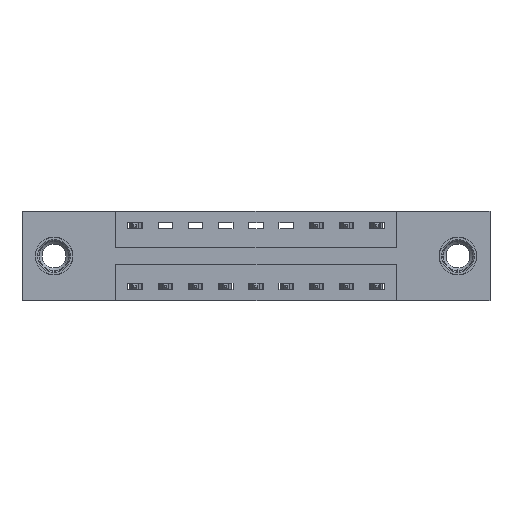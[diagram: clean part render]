
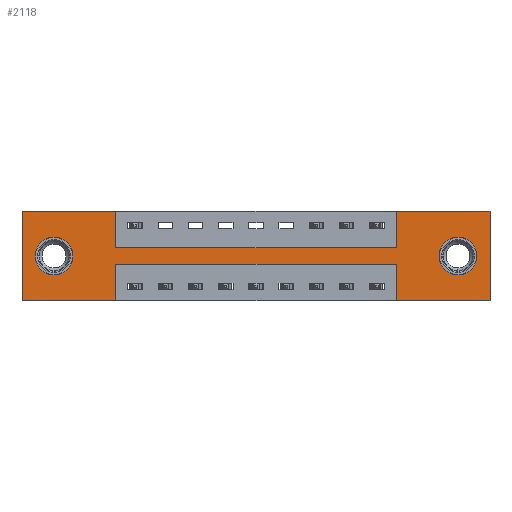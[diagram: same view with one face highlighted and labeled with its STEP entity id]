
A CAD part, front view. The second image highlights one B-rep face of the part: STEP entity #2118.
In plain terms, the highlighted planar face has unit normal (0, -1, 0).
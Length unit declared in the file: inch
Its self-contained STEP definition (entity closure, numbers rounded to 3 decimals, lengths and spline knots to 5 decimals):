
#57 = CARTESIAN_POINT ( 'NONE',  ( 1.935, 0., 0. ) ) ;
#127 = VECTOR ( 'NONE', #6239, 39.37008 ) ;
#150 = DIRECTION ( 'NONE',  ( 0., 1., 0. ) ) ;
#195 = VERTEX_POINT ( 'NONE', #1188 ) ;
#351 = DIRECTION ( 'NONE',  ( 0., 1., 0. ) ) ;
#354 = EDGE_CURVE ( 'NONE', #7185, #7598, #6876, .T. ) ;
#405 = FACE_BOUND ( 'NONE', #10598, .T. ) ;
#588 = ORIENTED_EDGE ( 'NONE', *, *, #4036, .T. ) ;
#617 = DIRECTION ( 'NONE',  ( -1., 0., 0. ) ) ;
#630 = VECTOR ( 'NONE', #2330, 39.37008 ) ;
#754 = VECTOR ( 'NONE', #3421, 39.37008 ) ;
#954 = CARTESIAN_POINT ( 'NONE',  ( 1.5475, 0., -0.37 ) ) ;
#1026 = LINE ( 'NONE', #11291, #754 ) ;
#1104 = ORIENTED_EDGE ( 'NONE', *, *, #2130, .F. ) ;
#1188 = CARTESIAN_POINT ( 'NONE',  ( 1.935, 0., -0.37 ) ) ;
#1241 = VECTOR ( 'NONE', #8316, 39.37008 ) ;
#1261 = VECTOR ( 'NONE', #5173, 39.37008 ) ;
#1417 = CARTESIAN_POINT ( 'NONE',  ( 1.8025, 0., -0.263 ) ) ;
#1550 = EDGE_CURVE ( 'NONE', #11316, #2201, #3587, .T. ) ;
#1667 = CARTESIAN_POINT ( 'NONE',  ( 0.3875, 0., 0. ) ) ;
#1832 = ORIENTED_EDGE ( 'NONE', *, *, #4395, .F. ) ;
#1946 = VECTOR ( 'NONE', #5117, 39.37008 ) ;
#2118 = ADVANCED_FACE ( 'NONE', ( #405, #2480, #7089 ), #8846, .T. ) ;
#2130 = EDGE_CURVE ( 'NONE', #7598, #3999, #9184, .T. ) ;
#2134 = VECTOR ( 'NONE', #10495, 39.37008 ) ;
#2201 = VERTEX_POINT ( 'NONE', #4592 ) ;
#2222 = CARTESIAN_POINT ( 'NONE',  ( 1.8025, 0., -0.107 ) ) ;
#2330 = DIRECTION ( 'NONE',  ( 1., 0., 0. ) ) ;
#2353 = CIRCLE ( 'NONE', #6170, 0.078 ) ;
#2410 = ORIENTED_EDGE ( 'NONE', *, *, #9981, .F. ) ;
#2420 = CIRCLE ( 'NONE', #6364, 0.078 ) ;
#2474 = DIRECTION ( 'NONE',  ( 1., 0., 0. ) ) ;
#2480 = FACE_BOUND ( 'NONE', #8097, .T. ) ;
#2612 = CARTESIAN_POINT ( 'NONE',  ( 0.3875, 0., -0.15 ) ) ;
#2656 = ORIENTED_EDGE ( 'NONE', *, *, #7369, .T. ) ;
#2743 = DIRECTION ( 'NONE',  ( 0., 1., 0. ) ) ;
#2757 = EDGE_CURVE ( 'NONE', #5667, #10404, #11383, .T. ) ;
#2888 = ORIENTED_EDGE ( 'NONE', *, *, #354, .F. ) ;
#2892 = CARTESIAN_POINT ( 'NONE',  ( 1.5475, 0., 0. ) ) ;
#2978 = VERTEX_POINT ( 'NONE', #9190 ) ;
#3146 = DIRECTION ( 'NONE',  ( 0., 0., 1. ) ) ;
#3162 = VERTEX_POINT ( 'NONE', #3290 ) ;
#3273 = ORIENTED_EDGE ( 'NONE', *, *, #5122, .F. ) ;
#3290 = CARTESIAN_POINT ( 'NONE',  ( 0.3875, 0., 0. ) ) ;
#3421 = DIRECTION ( 'NONE',  ( 0., 0., -1. ) ) ;
#3515 = AXIS2_PLACEMENT_3D ( 'NONE', #7959, #2743, #8843 ) ;
#3536 = EDGE_CURVE ( 'NONE', #6486, #195, #6248, .T. ) ;
#3587 = LINE ( 'NONE', #4345, #1241 ) ;
#3605 = DIRECTION ( 'NONE',  ( 0., 1., 0. ) ) ;
#3626 = CARTESIAN_POINT ( 'NONE',  ( 0., 0., -0.37 ) ) ;
#3650 = LINE ( 'NONE', #5843, #8001 ) ;
#3741 = DIRECTION ( 'NONE',  ( 0., 0., -1. ) ) ;
#3999 = VERTEX_POINT ( 'NONE', #6162 ) ;
#4036 = EDGE_CURVE ( 'NONE', #7563, #2978, #7182, .T. ) ;
#4074 = CARTESIAN_POINT ( 'NONE',  ( 1.5475, 0., -0.22 ) ) ;
#4232 = CARTESIAN_POINT ( 'NONE',  ( 0.3875, 0., -0.15 ) ) ;
#4345 = CARTESIAN_POINT ( 'NONE',  ( 0., 0., 0. ) ) ;
#4395 = EDGE_CURVE ( 'NONE', #2201, #3162, #5953, .T. ) ;
#4423 = LINE ( 'NONE', #7824, #2134 ) ;
#4437 = EDGE_CURVE ( 'NONE', #3999, #5343, #1026, .T. ) ;
#4473 = CARTESIAN_POINT ( 'NONE',  ( 0.3875, 0., -0.22 ) ) ;
#4592 = CARTESIAN_POINT ( 'NONE',  ( 0., 0., 0. ) ) ;
#5058 = ORIENTED_EDGE ( 'NONE', *, *, #6924, .F. ) ;
#5116 = CARTESIAN_POINT ( 'NONE',  ( 1.5475, 0., -0.15 ) ) ;
#5117 = DIRECTION ( 'NONE',  ( 1., 0., 0. ) ) ;
#5122 = EDGE_CURVE ( 'NONE', #195, #7185, #3650, .T. ) ;
#5173 = DIRECTION ( 'NONE',  ( 0., 0., -1. ) ) ;
#5343 = VERTEX_POINT ( 'NONE', #6151 ) ;
#5368 = DIRECTION ( 'NONE',  ( 0., 0., -1. ) ) ;
#5387 = AXIS2_PLACEMENT_3D ( 'NONE', #3626, #10645, #5368 ) ;
#5389 = CARTESIAN_POINT ( 'NONE',  ( 1.8025, 0., -0.185 ) ) ;
#5522 = DIRECTION ( 'NONE',  ( 0., 0., 1. ) ) ;
#5542 = AXIS2_PLACEMENT_3D ( 'NONE', #5389, #150, #6262 ) ;
#5581 = CARTESIAN_POINT ( 'NONE',  ( 1.8025, 0., -0.185 ) ) ;
#5597 = VECTOR ( 'NONE', #5522, 39.37008 ) ;
#5667 = VERTEX_POINT ( 'NONE', #1417 ) ;
#5743 = CARTESIAN_POINT ( 'NONE',  ( 0., 0., -0.37 ) ) ;
#5798 = CARTESIAN_POINT ( 'NONE',  ( 0.1325, 0., -0.263 ) ) ;
#5843 = CARTESIAN_POINT ( 'NONE',  ( 0., 0., -0.37 ) ) ;
#5921 = EDGE_CURVE ( 'NONE', #5343, #11316, #4423, .T. ) ;
#5953 = LINE ( 'NONE', #10357, #7999 ) ;
#6151 = CARTESIAN_POINT ( 'NONE',  ( 0.3875, 0., -0.37 ) ) ;
#6162 = CARTESIAN_POINT ( 'NONE',  ( 0.3875, 0., -0.22 ) ) ;
#6170 = AXIS2_PLACEMENT_3D ( 'NONE', #8825, #3605, #9724 ) ;
#6239 = DIRECTION ( 'NONE',  ( -1., 0., 0. ) ) ;
#6248 = LINE ( 'NONE', #9023, #10390 ) ;
#6262 = DIRECTION ( 'NONE',  ( 0., 0., -1. ) ) ;
#6364 = AXIS2_PLACEMENT_3D ( 'NONE', #5581, #351, #6455 ) ;
#6455 = DIRECTION ( 'NONE',  ( 0., 0., -1. ) ) ;
#6486 = VERTEX_POINT ( 'NONE', #57 ) ;
#6597 = VECTOR ( 'NONE', #3146, 39.37008 ) ;
#6793 = ORIENTED_EDGE ( 'NONE', *, *, #4437, .F. ) ;
#6876 = LINE ( 'NONE', #8363, #6597 ) ;
#6924 = EDGE_CURVE ( 'NONE', #8419, #6486, #7322, .T. ) ;
#7058 = ORIENTED_EDGE ( 'NONE', *, *, #9382, .F. ) ;
#7089 = FACE_OUTER_BOUND ( 'NONE', #10559, .T. ) ;
#7182 = CIRCLE ( 'NONE', #3515, 0.078 ) ;
#7185 = VERTEX_POINT ( 'NONE', #954 ) ;
#7322 = LINE ( 'NONE', #11103, #630 ) ;
#7369 = EDGE_CURVE ( 'NONE', #10404, #5667, #2420, .T. ) ;
#7563 = VERTEX_POINT ( 'NONE', #5798 ) ;
#7598 = VERTEX_POINT ( 'NONE', #4074 ) ;
#7707 = VERTEX_POINT ( 'NONE', #5116 ) ;
#7773 = VERTEX_POINT ( 'NONE', #2612 ) ;
#7824 = CARTESIAN_POINT ( 'NONE',  ( 0., 0., -0.37 ) ) ;
#7959 = CARTESIAN_POINT ( 'NONE',  ( 0.1325, 0., -0.185 ) ) ;
#7999 = VECTOR ( 'NONE', #2474, 39.37008 ) ;
#8001 = VECTOR ( 'NONE', #617, 39.37008 ) ;
#8097 = EDGE_LOOP ( 'NONE', ( #9697, #588 ) ) ;
#8316 = DIRECTION ( 'NONE',  ( 0., 0., 1. ) ) ;
#8363 = CARTESIAN_POINT ( 'NONE',  ( 1.5475, 0., -0.37 ) ) ;
#8419 = VERTEX_POINT ( 'NONE', #9970 ) ;
#8632 = LINE ( 'NONE', #4232, #1946 ) ;
#8825 = CARTESIAN_POINT ( 'NONE',  ( 0.1325, 0., -0.185 ) ) ;
#8843 = DIRECTION ( 'NONE',  ( 0., 0., 1. ) ) ;
#8846 = PLANE ( 'NONE',  #5387 ) ;
#9023 = CARTESIAN_POINT ( 'NONE',  ( 1.935, 0., 0. ) ) ;
#9184 = LINE ( 'NONE', #4473, #127 ) ;
#9190 = CARTESIAN_POINT ( 'NONE',  ( 0.1325, 0., -0.107 ) ) ;
#9382 = EDGE_CURVE ( 'NONE', #3162, #7773, #11152, .T. ) ;
#9540 = ORIENTED_EDGE ( 'NONE', *, *, #5921, .F. ) ;
#9697 = ORIENTED_EDGE ( 'NONE', *, *, #10146, .T. ) ;
#9724 = DIRECTION ( 'NONE',  ( 0., 0., 1. ) ) ;
#9970 = CARTESIAN_POINT ( 'NONE',  ( 1.5475, 0., 0. ) ) ;
#9981 = EDGE_CURVE ( 'NONE', #7773, #7707, #8632, .T. ) ;
#10146 = EDGE_CURVE ( 'NONE', #2978, #7563, #2353, .T. ) ;
#10170 = ORIENTED_EDGE ( 'NONE', *, *, #11155, .F. ) ;
#10247 = ORIENTED_EDGE ( 'NONE', *, *, #1550, .F. ) ;
#10357 = CARTESIAN_POINT ( 'NONE',  ( 0., 0., 0. ) ) ;
#10390 = VECTOR ( 'NONE', #3741, 39.37008 ) ;
#10404 = VERTEX_POINT ( 'NONE', #2222 ) ;
#10495 = DIRECTION ( 'NONE',  ( -1., 0., 0. ) ) ;
#10559 = EDGE_LOOP ( 'NONE', ( #6793, #1104, #2888, #3273, #10608, #5058, #10170, #2410, #7058, #1832, #10247, #9540 ) ) ;
#10598 = EDGE_LOOP ( 'NONE', ( #2656, #10798 ) ) ;
#10608 = ORIENTED_EDGE ( 'NONE', *, *, #3536, .F. ) ;
#10645 = DIRECTION ( 'NONE',  ( 0., -1., 0. ) ) ;
#10798 = ORIENTED_EDGE ( 'NONE', *, *, #2757, .T. ) ;
#11103 = CARTESIAN_POINT ( 'NONE',  ( 0., 0., 0. ) ) ;
#11108 = LINE ( 'NONE', #2892, #5597 ) ;
#11152 = LINE ( 'NONE', #1667, #1261 ) ;
#11155 = EDGE_CURVE ( 'NONE', #7707, #8419, #11108, .T. ) ;
#11291 = CARTESIAN_POINT ( 'NONE',  ( 0.3875, 0., -0.37 ) ) ;
#11316 = VERTEX_POINT ( 'NONE', #5743 ) ;
#11383 = CIRCLE ( 'NONE', #5542, 0.078 ) ;
